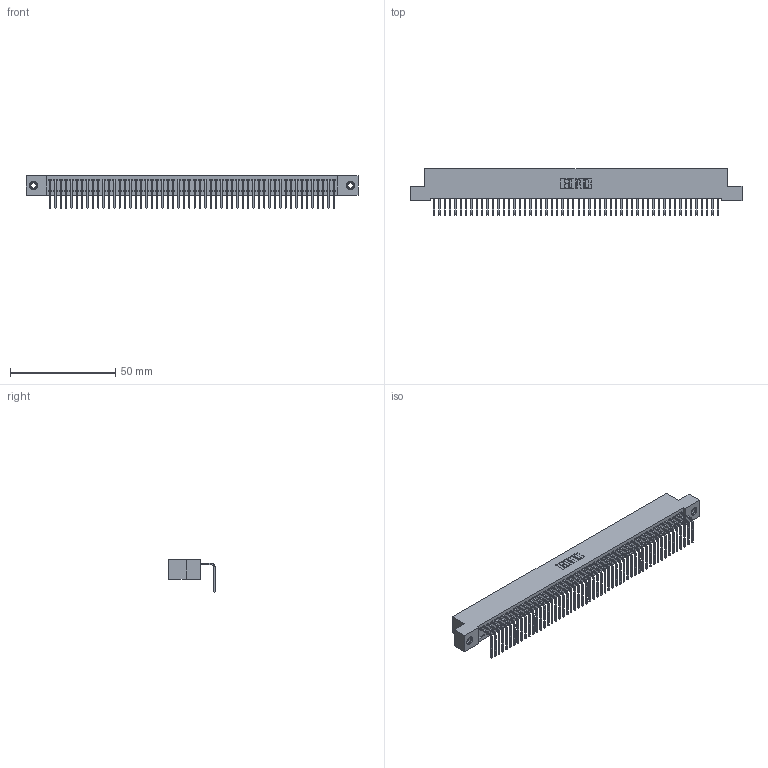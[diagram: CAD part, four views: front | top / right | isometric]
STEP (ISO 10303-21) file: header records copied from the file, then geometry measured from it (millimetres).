
FILE_DESCRIPTION (( 'STEP AP203' ), '1' );
FILE_NAME ('392-054-558-107.STEP', '2019-10-08T14:07:08', ( '' ), ( '' ), 'SwSTEP 2.0', 'SolidWorks 2016', '' );
FILE_SCHEMA (( 'CONFIG_CONTROL_DESIGN' ));
Length unit declared in the file: inch
Products named in the file (4): 345-292-001_558 Tail - 2; 345-250-001_345-250-005-103; 392-054-558-107; 342 Part_TI
Assembly tree (57 placements, depth 2):
  392-054-558-107
    342 Part_TI
    345-292-001_558 Tail - 2  x54
    345-250-001_345-250-005-103  x2
Bounding box: 157.48 x 21.91 x 15.62 mm (x, y, z)
Volume: 14019.3 mm3; surface area: 21864.7 mm2
Topology: 57 solids, 57 shells, 3410 faces, 10263 edges, 6762 vertices
Faces by surface type: plane 2474, cylinder 920, cone 12, torus 4
Entity records: 32598 total; most frequent: CARTESIAN_POINT 5603, ORIENTED_EDGE 5586, DIRECTION 4735, EDGE_CURVE 2793, VECTOR 2645, LINE 2645, VERTEX_POINT 1856, AXIS2_PLACEMENT_3D 1045
